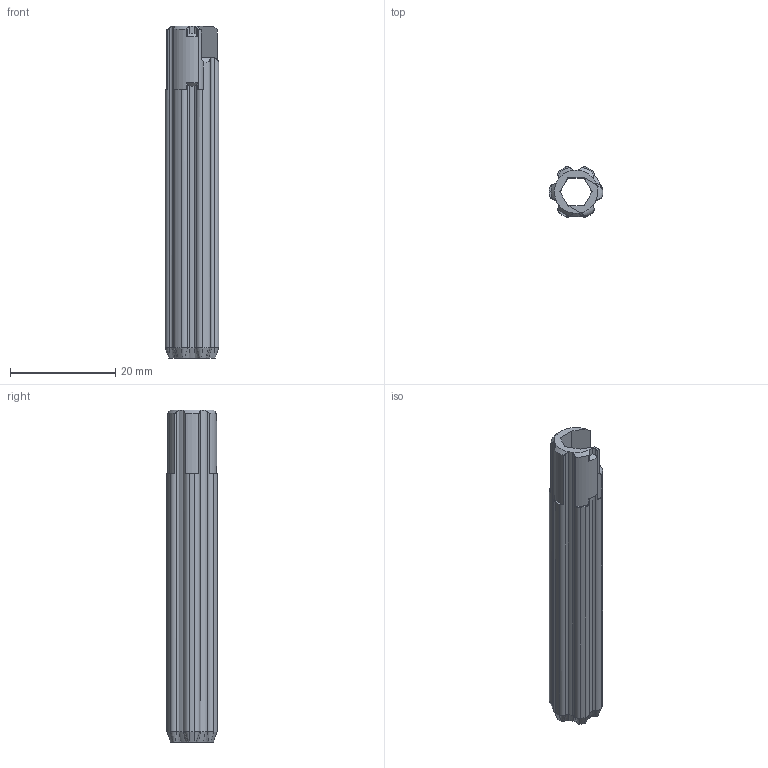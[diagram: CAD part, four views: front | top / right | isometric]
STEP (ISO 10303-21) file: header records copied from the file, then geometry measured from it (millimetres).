
FILE_DESCRIPTION(/* description */ (''),/* implementation_level */ '2;1');
FILE_NAME(/* name */ 'Charging Handle Bushing.step',/* time_stamp */ '2022-05-11T21:17:38-06:00',/* author */ (''),/* organization */ (''),/* preprocessor_version */ 'ST-DEVELOPER v18.1',/* originating_system */ 'Autodesk Translation Framework v10.10.0.1391',/* authorisation */ '');
FILE_SCHEMA (('AUTOMOTIVE_DESIGN { 1 0 10303 214 3 1 1 }'));
Length unit declared in the file: millimetre
Products named in the file (1): Charging Handle Bushing
Bounding box: 10.2 x 9.51 x 62.97 mm (x, y, z)
Volume: 2686 mm3; surface area: 3287.2 mm2
Topology: 1 solids, 1 shells, 121 faces, 312 edges, 192 vertices
Faces by surface type: cylinder 52, cone 46, plane 21, torus 2
Entity records: 3860 total; most frequent: CARTESIAN_POINT 884, DIRECTION 634, ORIENTED_EDGE 624, EDGE_CURVE 312, AXIS2_PLACEMENT_3D 260, VERTEX_POINT 192, CIRCLE 138, EDGE_LOOP 122
